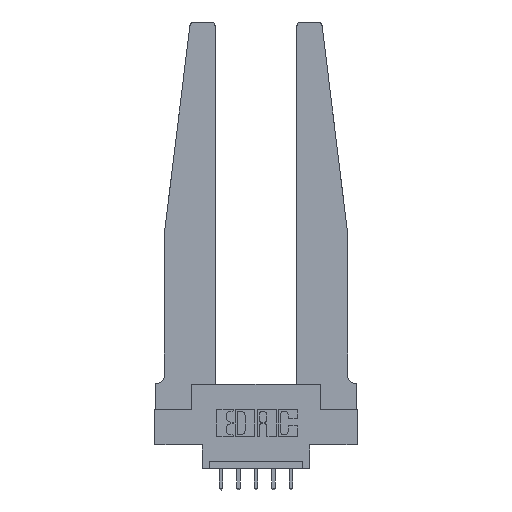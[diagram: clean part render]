
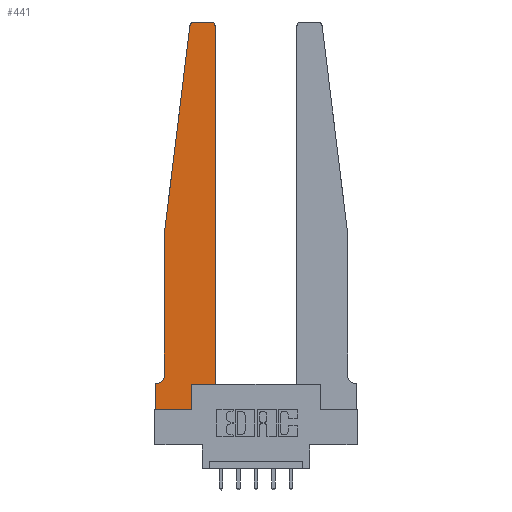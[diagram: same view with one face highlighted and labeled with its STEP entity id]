
A CAD part, top view. The second image highlights one B-rep face of the part: STEP entity #441.
In plain terms, the highlighted planar face has unit normal (0, 0, 1).
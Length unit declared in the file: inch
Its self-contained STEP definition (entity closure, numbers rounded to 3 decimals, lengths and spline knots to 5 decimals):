
#441 = ADVANCED_FACE ( 'NONE', ( #10658 ), #11059, .T. ) ;
#443 = ORIENTED_EDGE ( 'NONE', *, *, #3643, .T. ) ;
#463 = VERTEX_POINT ( 'NONE', #1581 ) ;
#696 = VERTEX_POINT ( 'NONE', #819 ) ;
#705 = VECTOR ( 'NONE', #9448, 39.37008 ) ;
#748 = CARTESIAN_POINT ( 'NONE',  ( 0.015, 0.1875, 0.37 ) ) ;
#802 = VERTEX_POINT ( 'NONE', #1094 ) ;
#819 = CARTESIAN_POINT ( 'NONE',  ( 0., 0.1875, 0.37 ) ) ;
#836 = CARTESIAN_POINT ( 'NONE',  ( 0., 0., 0.37 ) ) ;
#914 = ORIENTED_EDGE ( 'NONE', *, *, #11864, .T. ) ;
#1051 = LINE ( 'NONE', #2069, #3551 ) ;
#1094 = CARTESIAN_POINT ( 'NONE',  ( 0.425, 2.72, 0.37 ) ) ;
#1192 = CARTESIAN_POINT ( 'NONE',  ( 0.425, 0.18, 0.37 ) ) ;
#1386 = EDGE_LOOP ( 'NONE', ( #3805, #12187, #4628, #914, #5689, #9127, #4817, #8526, #4199, #12761, #4005, #443 ) ) ;
#1407 = VECTOR ( 'NONE', #4554, 39.37008 ) ;
#1431 = LINE ( 'NONE', #2310, #10845 ) ;
#1581 = CARTESIAN_POINT ( 'NONE',  ( 0.2605, 0., 0.37 ) ) ;
#1663 = DIRECTION ( 'NONE',  ( 1., 0., 0. ) ) ;
#1767 = DIRECTION ( 'NONE',  ( -1., 0., 0. ) ) ;
#1886 = CARTESIAN_POINT ( 'NONE',  ( 0.2605, 0.18, 0.37 ) ) ;
#1907 = DIRECTION ( 'NONE',  ( 0., 0., 1. ) ) ;
#2069 = CARTESIAN_POINT ( 'NONE',  ( 0.425, 0.18, 0.37 ) ) ;
#2208 = CARTESIAN_POINT ( 'NONE',  ( 0., 0., 0.37 ) ) ;
#2310 = CARTESIAN_POINT ( 'NONE',  ( 0.065, 1.25, 0.37 ) ) ;
#2360 = CARTESIAN_POINT ( 'NONE',  ( 0., 0., 0.37 ) ) ;
#2899 = AXIS2_PLACEMENT_3D ( 'NONE', #5662, #4673, #12051 ) ;
#2918 = VECTOR ( 'NONE', #11309, 39.37008 ) ;
#2974 = CIRCLE ( 'NONE', #10510, 0.05 ) ;
#3357 = DIRECTION ( 'NONE',  ( 1., 0., 0. ) ) ;
#3460 = DIRECTION ( 'NONE',  ( -0.122, -0.992, 0. ) ) ;
#3551 = VECTOR ( 'NONE', #3357, 39.37008 ) ;
#3643 = EDGE_CURVE ( 'NONE', #802, #11017, #8486, .T. ) ;
#3805 = ORIENTED_EDGE ( 'NONE', *, *, #10026, .T. ) ;
#3841 = CARTESIAN_POINT ( 'NONE',  ( 0.27653, 2.72, 0.37 ) ) ;
#3865 = VECTOR ( 'NONE', #4461, 39.37008 ) ;
#4005 = ORIENTED_EDGE ( 'NONE', *, *, #8131, .T. ) ;
#4129 = DIRECTION ( 'NONE',  ( 1., 0., 0. ) ) ;
#4199 = ORIENTED_EDGE ( 'NONE', *, *, #9237, .T. ) ;
#4302 = VERTEX_POINT ( 'NONE', #6041 ) ;
#4461 = DIRECTION ( 'NONE',  ( -1., 0., 0. ) ) ;
#4554 = DIRECTION ( 'NONE',  ( 0., -1., 0. ) ) ;
#4628 = ORIENTED_EDGE ( 'NONE', *, *, #7207, .T. ) ;
#4673 = DIRECTION ( 'NONE',  ( 0., 0., 1. ) ) ;
#4817 = ORIENTED_EDGE ( 'NONE', *, *, #10389, .T. ) ;
#4941 = LINE ( 'NONE', #836, #8805 ) ;
#4984 = VERTEX_POINT ( 'NONE', #12238 ) ;
#5008 = VERTEX_POINT ( 'NONE', #9730 ) ;
#5038 = LINE ( 'NONE', #1886, #2918 ) ;
#5059 = DIRECTION ( 'NONE',  ( 1., 0., 0. ) ) ;
#5662 = CARTESIAN_POINT ( 'NONE',  ( 0., 0.1875, 0.37 ) ) ;
#5689 = ORIENTED_EDGE ( 'NONE', *, *, #11150, .T. ) ;
#6041 = CARTESIAN_POINT ( 'NONE',  ( 0.425, 0.18, 0.37 ) ) ;
#6277 = CARTESIAN_POINT ( 'NONE',  ( 0.015, 0.2375, 0.37 ) ) ;
#6347 = AXIS2_PLACEMENT_3D ( 'NONE', #3841, #1907, #5059 ) ;
#6482 = VERTEX_POINT ( 'NONE', #2208 ) ;
#7207 = EDGE_CURVE ( 'NONE', #10585, #8362, #1431, .T. ) ;
#7211 = DIRECTION ( 'NONE',  ( 0., -1., 0. ) ) ;
#7414 = DIRECTION ( 'NONE',  ( 0., 0., -1. ) ) ;
#7858 = CARTESIAN_POINT ( 'NONE',  ( 0.25, 2.75, 0.37 ) ) ;
#7985 = CARTESIAN_POINT ( 'NONE',  ( 0.065, 1.25, 0.37 ) ) ;
#8131 = EDGE_CURVE ( 'NONE', #4302, #802, #11422, .T. ) ;
#8149 = VECTOR ( 'NONE', #7211, 39.37008 ) ;
#8282 = DIRECTION ( 'NONE',  ( 0., 0., 1. ) ) ;
#8362 = VERTEX_POINT ( 'NONE', #7985 ) ;
#8486 = CIRCLE ( 'NONE', #12639, 0.03 ) ;
#8489 = LINE ( 'NONE', #9552, #3865 ) ;
#8526 = ORIENTED_EDGE ( 'NONE', *, *, #12949, .T. ) ;
#8604 = CARTESIAN_POINT ( 'NONE',  ( 0.065, 0.2375, 0.37 ) ) ;
#8805 = VECTOR ( 'NONE', #1663, 39.37008 ) ;
#9127 = ORIENTED_EDGE ( 'NONE', *, *, #12181, .T. ) ;
#9237 = EDGE_CURVE ( 'NONE', #463, #5008, #5038, .T. ) ;
#9309 = CARTESIAN_POINT ( 'NONE',  ( 0.24675, 2.72367, 0.37 ) ) ;
#9448 = DIRECTION ( 'NONE',  ( 0., 1., 0. ) ) ;
#9552 = CARTESIAN_POINT ( 'NONE',  ( 0.065, 0.1875, 0.37 ) ) ;
#9730 = CARTESIAN_POINT ( 'NONE',  ( 0.2605, 0.18, 0.37 ) ) ;
#9895 = EDGE_CURVE ( 'NONE', #5008, #4302, #1051, .T. ) ;
#10026 = EDGE_CURVE ( 'NONE', #11017, #4984, #10727, .T. ) ;
#10084 = EDGE_CURVE ( 'NONE', #4984, #10585, #12862, .T. ) ;
#10170 = CARTESIAN_POINT ( 'NONE',  ( 0.395, 2.72, 0.37 ) ) ;
#10389 = EDGE_CURVE ( 'NONE', #696, #6482, #10461, .T. ) ;
#10447 = LINE ( 'NONE', #10528, #8149 ) ;
#10461 = LINE ( 'NONE', #2360, #1407 ) ;
#10510 = AXIS2_PLACEMENT_3D ( 'NONE', #6277, #7414, #13369 ) ;
#10528 = CARTESIAN_POINT ( 'NONE',  ( 0.065, 1.25, 0.37 ) ) ;
#10585 = VERTEX_POINT ( 'NONE', #9309 ) ;
#10658 = FACE_OUTER_BOUND ( 'NONE', #1386, .T. ) ;
#10727 = LINE ( 'NONE', #7858, #11803 ) ;
#10845 = VECTOR ( 'NONE', #3460, 39.37008 ) ;
#11017 = VERTEX_POINT ( 'NONE', #13292 ) ;
#11059 = PLANE ( 'NONE',  #2899 ) ;
#11150 = EDGE_CURVE ( 'NONE', #12531, #12633, #2974, .T. ) ;
#11309 = DIRECTION ( 'NONE',  ( 0., 1., 0. ) ) ;
#11422 = LINE ( 'NONE', #1192, #705 ) ;
#11803 = VECTOR ( 'NONE', #1767, 39.37008 ) ;
#11864 = EDGE_CURVE ( 'NONE', #8362, #12531, #10447, .T. ) ;
#12051 = DIRECTION ( 'NONE',  ( 1., 0., 0. ) ) ;
#12181 = EDGE_CURVE ( 'NONE', #12633, #696, #8489, .T. ) ;
#12187 = ORIENTED_EDGE ( 'NONE', *, *, #10084, .T. ) ;
#12238 = CARTESIAN_POINT ( 'NONE',  ( 0.27653, 2.75, 0.37 ) ) ;
#12531 = VERTEX_POINT ( 'NONE', #8604 ) ;
#12633 = VERTEX_POINT ( 'NONE', #748 ) ;
#12639 = AXIS2_PLACEMENT_3D ( 'NONE', #10170, #8282, #4129 ) ;
#12761 = ORIENTED_EDGE ( 'NONE', *, *, #9895, .T. ) ;
#12862 = CIRCLE ( 'NONE', #6347, 0.03 ) ;
#12949 = EDGE_CURVE ( 'NONE', #6482, #463, #4941, .T. ) ;
#13292 = CARTESIAN_POINT ( 'NONE',  ( 0.395, 2.75, 0.37 ) ) ;
#13369 = DIRECTION ( 'NONE',  ( -1., 0., 0. ) ) ;
